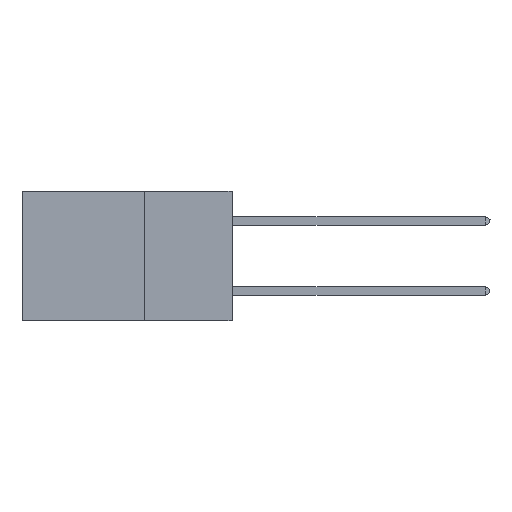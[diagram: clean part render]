
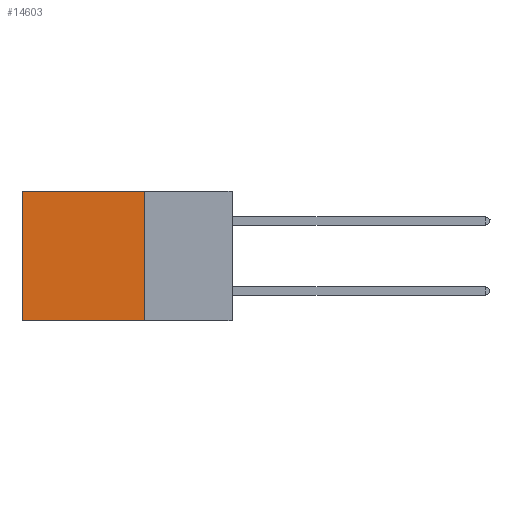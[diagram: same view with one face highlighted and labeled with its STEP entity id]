
A CAD part, left-side view. The second image highlights one B-rep face of the part: STEP entity #14603.
In plain terms, the highlighted planar face has unit normal (-1, 0, 0).
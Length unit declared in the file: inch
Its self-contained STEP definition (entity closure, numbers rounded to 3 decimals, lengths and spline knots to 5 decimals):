
#67 = CARTESIAN_POINT ( 'NONE',  ( 0.2875, 0.6, 0. ) ) ;
#843 = ORIENTED_EDGE ( 'NONE', *, *, #10169, .T. ) ;
#2211 = VECTOR ( 'NONE', #11056, 39.37008 ) ;
#2642 = VERTEX_POINT ( 'NONE', #20554 ) ;
#4293 = CARTESIAN_POINT ( 'NONE',  ( 0.2875, 0.25, 0. ) ) ;
#4385 = DIRECTION ( 'NONE',  ( 0., 0., -1. ) ) ;
#7369 = EDGE_CURVE ( 'NONE', #2642, #27256, #22406, .T. ) ;
#8147 = VERTEX_POINT ( 'NONE', #17366 ) ;
#9821 = VECTOR ( 'NONE', #27669, 39.37008 ) ;
#9971 = CARTESIAN_POINT ( 'NONE',  ( 0.2875, 0.25, -0.37 ) ) ;
#10169 = EDGE_CURVE ( 'NONE', #14277, #27256, #15944, .T. ) ;
#10315 = DIRECTION ( 'NONE',  ( 0., 0., -1. ) ) ;
#11056 = DIRECTION ( 'NONE',  ( 0., 1., 0. ) ) ;
#14277 = VERTEX_POINT ( 'NONE', #21247 ) ;
#14603 = ADVANCED_FACE ( 'NONE', ( #20773 ), #24529, .F. ) ;
#15001 = ORIENTED_EDGE ( 'NONE', *, *, #28230, .T. ) ;
#15944 = LINE ( 'NONE', #67, #26966 ) ;
#16150 = ORIENTED_EDGE ( 'NONE', *, *, #7369, .F. ) ;
#16326 = EDGE_CURVE ( 'NONE', #8147, #2642, #23783, .T. ) ;
#17366 = CARTESIAN_POINT ( 'NONE',  ( 0.2875, 0.25, 0. ) ) ;
#17983 = DIRECTION ( 'NONE',  ( 1., 0., 0. ) ) ;
#18352 = DIRECTION ( 'NONE',  ( 0., 0., -1. ) ) ;
#18882 = CARTESIAN_POINT ( 'NONE',  ( 0.2875, 0.6, -0.37 ) ) ;
#19462 = AXIS2_PLACEMENT_3D ( 'NONE', #4293, #17983, #4385 ) ;
#20554 = CARTESIAN_POINT ( 'NONE',  ( 0.2875, 0.25, -0.37 ) ) ;
#20773 = FACE_OUTER_BOUND ( 'NONE', #27065, .T. ) ;
#21247 = CARTESIAN_POINT ( 'NONE',  ( 0.2875, 0.6, 0. ) ) ;
#22406 = LINE ( 'NONE', #9971, #9821 ) ;
#23104 = VECTOR ( 'NONE', #10315, 39.37008 ) ;
#23783 = LINE ( 'NONE', #28009, #23104 ) ;
#24529 = PLANE ( 'NONE',  #19462 ) ;
#25459 = LINE ( 'NONE', #28729, #2211 ) ;
#26966 = VECTOR ( 'NONE', #18352, 39.37008 ) ;
#27065 = EDGE_LOOP ( 'NONE', ( #843, #16150, #28803, #15001 ) ) ;
#27256 = VERTEX_POINT ( 'NONE', #18882 ) ;
#27669 = DIRECTION ( 'NONE',  ( 0., 1., 0. ) ) ;
#28009 = CARTESIAN_POINT ( 'NONE',  ( 0.2875, 0.25, 0. ) ) ;
#28230 = EDGE_CURVE ( 'NONE', #8147, #14277, #25459, .T. ) ;
#28729 = CARTESIAN_POINT ( 'NONE',  ( 0.2875, 0.25, 0. ) ) ;
#28803 = ORIENTED_EDGE ( 'NONE', *, *, #16326, .F. ) ;
